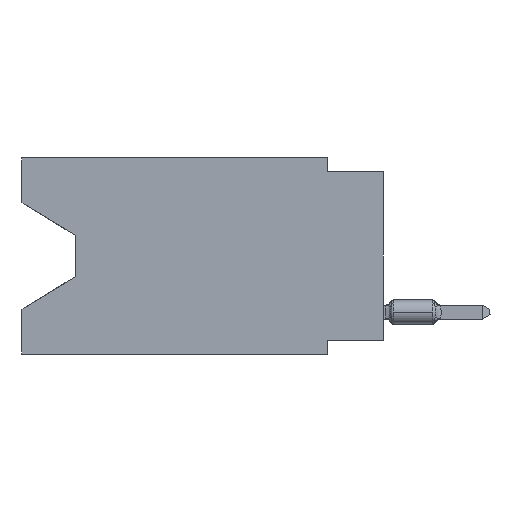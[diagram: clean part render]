
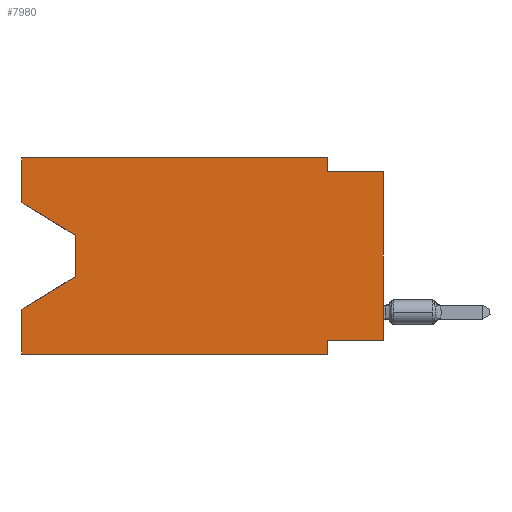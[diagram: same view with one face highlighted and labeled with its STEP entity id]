
A CAD part, left-side view. The second image highlights one B-rep face of the part: STEP entity #7980.
In plain terms, the highlighted planar face has unit normal (-1, 0, 0).
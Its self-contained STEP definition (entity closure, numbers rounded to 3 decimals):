
#448 = CARTESIAN_POINT ( 'NONE',  ( 0., 16.383, 0. ) ) ;
#517 = DIRECTION ( 'NONE',  ( 0., 0.855, -0.519 ) ) ;
#940 = CARTESIAN_POINT ( 'NONE',  ( 0., 2.54, -8.89 ) ) ;
#1103 = DIRECTION ( 'NONE',  ( 0., 0., -1. ) ) ;
#2306 = CARTESIAN_POINT ( 'NONE',  ( 0., 13.97, -3.505 ) ) ;
#2312 = CARTESIAN_POINT ( 'NONE',  ( 0., 0., -8.255 ) ) ;
#3003 = LINE ( 'NONE', #16424, #9787 ) ;
#3528 = ORIENTED_EDGE ( 'NONE', *, *, #29955, .T. ) ;
#3659 = VERTEX_POINT ( 'NONE', #34011 ) ;
#4437 = CARTESIAN_POINT ( 'NONE',  ( 0., 2.54, 0. ) ) ;
#5266 = EDGE_LOOP ( 'NONE', ( #13264, #20952, #3528, #7299, #23943, #6541, #6094, #10827, #33642, #24159, #10887, #28509 ) ) ;
#5281 = VECTOR ( 'NONE', #22177, 1000. ) ;
#5442 = LINE ( 'NONE', #10844, #27648 ) ;
#5480 = LINE ( 'NONE', #16140, #33975 ) ;
#6074 = CARTESIAN_POINT ( 'NONE',  ( 0., 13.97, -5.385 ) ) ;
#6094 = ORIENTED_EDGE ( 'NONE', *, *, #22992, .F. ) ;
#6305 = LINE ( 'NONE', #21864, #13642 ) ;
#6312 = FACE_OUTER_BOUND ( 'NONE', #5266, .T. ) ;
#6358 = EDGE_CURVE ( 'NONE', #33151, #26977, #3003, .T. ) ;
#6541 = ORIENTED_EDGE ( 'NONE', *, *, #26969, .F. ) ;
#6544 = VERTEX_POINT ( 'NONE', #9590 ) ;
#6857 = DIRECTION ( 'NONE',  ( 0., -1., 0. ) ) ;
#7299 = ORIENTED_EDGE ( 'NONE', *, *, #30592, .F. ) ;
#7980 = ADVANCED_FACE ( 'NONE', ( #6312 ), #16968, .F. ) ;
#8568 = VECTOR ( 'NONE', #6857, 1000. ) ;
#8689 = LINE ( 'NONE', #6074, #23298 ) ;
#9582 = CARTESIAN_POINT ( 'NONE',  ( 0., 16.383, -2.038 ) ) ;
#9590 = CARTESIAN_POINT ( 'NONE',  ( 0., 16.383, -6.852 ) ) ;
#9787 = VECTOR ( 'NONE', #10839, 1000. ) ;
#10005 = LINE ( 'NONE', #4437, #18563 ) ;
#10462 = EDGE_CURVE ( 'NONE', #19780, #21121, #20148, .T. ) ;
#10679 = EDGE_CURVE ( 'NONE', #29004, #24554, #6305, .T. ) ;
#10827 = ORIENTED_EDGE ( 'NONE', *, *, #17427, .T. ) ;
#10839 = DIRECTION ( 'NONE',  ( 0., 0., -1. ) ) ;
#10844 = CARTESIAN_POINT ( 'NONE',  ( 0., 0., -8.255 ) ) ;
#10881 = DIRECTION ( 'NONE',  ( 0., 0., -1. ) ) ;
#10887 = ORIENTED_EDGE ( 'NONE', *, *, #10679, .F. ) ;
#11077 = DIRECTION ( 'NONE',  ( 0., 0., 1. ) ) ;
#11322 = EDGE_CURVE ( 'NONE', #33606, #33151, #22685, .T. ) ;
#13264 = ORIENTED_EDGE ( 'NONE', *, *, #11322, .T. ) ;
#13642 = VECTOR ( 'NONE', #14178, 1000. ) ;
#14178 = DIRECTION ( 'NONE',  ( 0., -1., 0. ) ) ;
#14844 = CARTESIAN_POINT ( 'NONE',  ( 0., 0., -0.635 ) ) ;
#16140 = CARTESIAN_POINT ( 'NONE',  ( 0., 2.54, -8.89 ) ) ;
#16341 = VECTOR ( 'NONE', #28439, 1000. ) ;
#16424 = CARTESIAN_POINT ( 'NONE',  ( 0., 13.97, -3.505 ) ) ;
#16505 = EDGE_CURVE ( 'NONE', #33606, #29004, #24373, .T. ) ;
#16736 = EDGE_CURVE ( 'NONE', #24554, #3659, #10005, .T. ) ;
#16968 = PLANE ( 'NONE',  #26098 ) ;
#17139 = DIRECTION ( 'NONE',  ( 1., 0., 0. ) ) ;
#17427 = EDGE_CURVE ( 'NONE', #34271, #23042, #25813, .T. ) ;
#18439 = CARTESIAN_POINT ( 'NONE',  ( 0., 0., 0. ) ) ;
#18461 = CARTESIAN_POINT ( 'NONE',  ( 0., 16.383, -8.89 ) ) ;
#18563 = VECTOR ( 'NONE', #33965, 1000. ) ;
#19780 = VERTEX_POINT ( 'NONE', #18461 ) ;
#20148 = LINE ( 'NONE', #30819, #8568 ) ;
#20870 = CARTESIAN_POINT ( 'NONE',  ( 0., 2.54, 0. ) ) ;
#20952 = ORIENTED_EDGE ( 'NONE', *, *, #6358, .T. ) ;
#21121 = VERTEX_POINT ( 'NONE', #940 ) ;
#21864 = CARTESIAN_POINT ( 'NONE',  ( 0., 16.383, 0. ) ) ;
#22177 = DIRECTION ( 'NONE',  ( 0., -0.855, -0.519 ) ) ;
#22685 = LINE ( 'NONE', #9582, #5281 ) ;
#22992 = EDGE_CURVE ( 'NONE', #34271, #29406, #5442, .T. ) ;
#23042 = VERTEX_POINT ( 'NONE', #14844 ) ;
#23298 = VECTOR ( 'NONE', #517, 1000. ) ;
#23395 = CARTESIAN_POINT ( 'NONE',  ( 0., 0., -0.635 ) ) ;
#23799 = DIRECTION ( 'NONE',  ( 0., 0., 1. ) ) ;
#23943 = ORIENTED_EDGE ( 'NONE', *, *, #10462, .T. ) ;
#24159 = ORIENTED_EDGE ( 'NONE', *, *, #16736, .F. ) ;
#24373 = LINE ( 'NONE', #448, #25248 ) ;
#24554 = VERTEX_POINT ( 'NONE', #20870 ) ;
#25028 = CARTESIAN_POINT ( 'NONE',  ( 0., 16.383, 0. ) ) ;
#25248 = VECTOR ( 'NONE', #11077, 1000. ) ;
#25813 = LINE ( 'NONE', #18439, #16341 ) ;
#25990 = CARTESIAN_POINT ( 'NONE',  ( 0., 16.383, 0. ) ) ;
#26098 = AXIS2_PLACEMENT_3D ( 'NONE', #25028, #17139, #1103 ) ;
#26940 = DIRECTION ( 'NONE',  ( 0., 1., 0. ) ) ;
#26969 = EDGE_CURVE ( 'NONE', #29406, #21121, #5480, .T. ) ;
#26977 = VERTEX_POINT ( 'NONE', #32225 ) ;
#27256 = VECTOR ( 'NONE', #23799, 1000. ) ;
#27648 = VECTOR ( 'NONE', #26940, 1000. ) ;
#28304 = LINE ( 'NONE', #23395, #29366 ) ;
#28439 = DIRECTION ( 'NONE',  ( 0., 0., 1. ) ) ;
#28509 = ORIENTED_EDGE ( 'NONE', *, *, #16505, .F. ) ;
#28888 = CARTESIAN_POINT ( 'NONE',  ( 0., 16.383, 0. ) ) ;
#29004 = VERTEX_POINT ( 'NONE', #25990 ) ;
#29366 = VECTOR ( 'NONE', #33879, 1000. ) ;
#29406 = VERTEX_POINT ( 'NONE', #30066 ) ;
#29955 = EDGE_CURVE ( 'NONE', #26977, #6544, #8689, .T. ) ;
#30066 = CARTESIAN_POINT ( 'NONE',  ( 0., 2.54, -8.255 ) ) ;
#30592 = EDGE_CURVE ( 'NONE', #19780, #6544, #34119, .T. ) ;
#30819 = CARTESIAN_POINT ( 'NONE',  ( 0., 16.383, -8.89 ) ) ;
#32225 = CARTESIAN_POINT ( 'NONE',  ( 0., 13.97, -5.385 ) ) ;
#32461 = CARTESIAN_POINT ( 'NONE',  ( 0., 16.383, -2.038 ) ) ;
#33151 = VERTEX_POINT ( 'NONE', #2306 ) ;
#33606 = VERTEX_POINT ( 'NONE', #32461 ) ;
#33642 = ORIENTED_EDGE ( 'NONE', *, *, #34512, .F. ) ;
#33879 = DIRECTION ( 'NONE',  ( 0., -1., 0. ) ) ;
#33965 = DIRECTION ( 'NONE',  ( 0., 0., -1. ) ) ;
#33975 = VECTOR ( 'NONE', #10881, 1000. ) ;
#34011 = CARTESIAN_POINT ( 'NONE',  ( 0., 2.54, -0.635 ) ) ;
#34119 = LINE ( 'NONE', #28888, #27256 ) ;
#34271 = VERTEX_POINT ( 'NONE', #2312 ) ;
#34512 = EDGE_CURVE ( 'NONE', #3659, #23042, #28304, .T. ) ;
